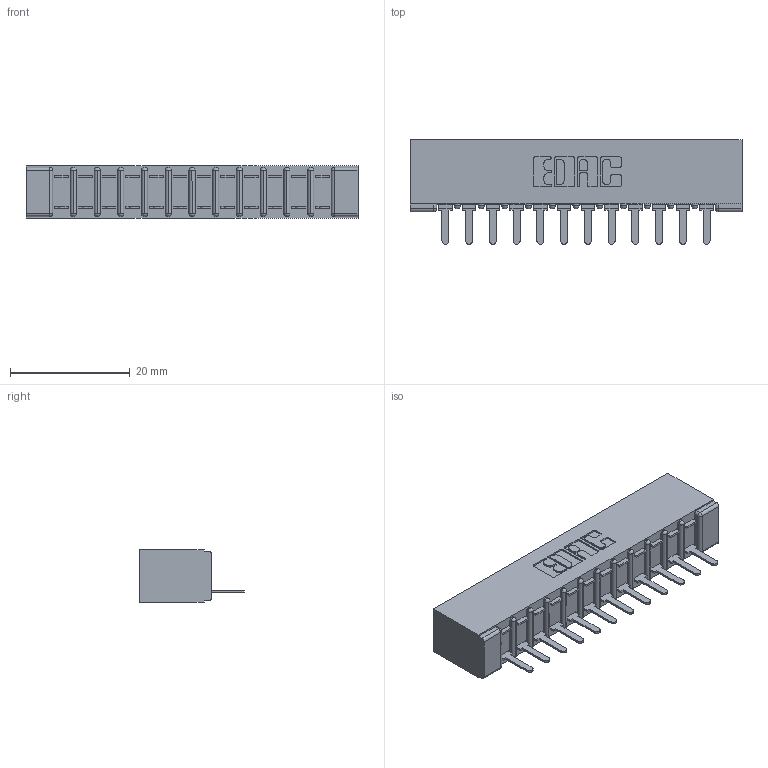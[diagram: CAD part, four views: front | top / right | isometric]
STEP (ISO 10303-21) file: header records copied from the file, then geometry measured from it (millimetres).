
FILE_DESCRIPTION (( 'STEP AP203' ), '1' );
FILE_NAME ('357-012-421-101.STEP', '2020-09-30T12:04:40', ( '' ), ( '' ), 'SwSTEP 2.0', 'SolidWorks 2020', '' );
FILE_SCHEMA (( 'CONFIG_CONTROL_DESIGN' ));
Length unit declared in the file: inch
Products named in the file (3): 307-290-002_521; 357-012-421-101; 307 Part_No Mounting Lugs
Assembly tree (13 placements, depth 2):
  357-012-421-101
    307 Part_No Mounting Lugs
    307-290-002_521  x12
Bounding box: 55.42 x 17.42 x 8.71 mm (x, y, z)
Volume: 3896.7 mm3; surface area: 7045.8 mm2
Topology: 13 solids, 13 shells, 1011 faces, 3083 edges, 2018 vertices
Faces by surface type: plane 606, cylinder 379, sphere 26
Entity records: 14426 total; most frequent: CARTESIAN_POINT 2428, ORIENTED_EDGE 2418, DIRECTION 2371, EDGE_CURVE 1209, LINE 913, VECTOR 913, VERTEX_POINT 786, AXIS2_PLACEMENT_3D 729
